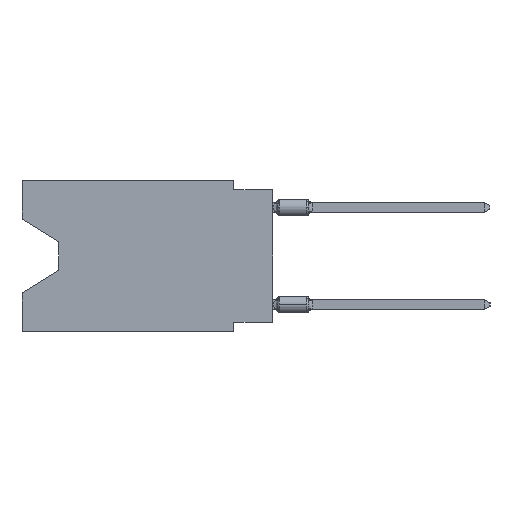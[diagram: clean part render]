
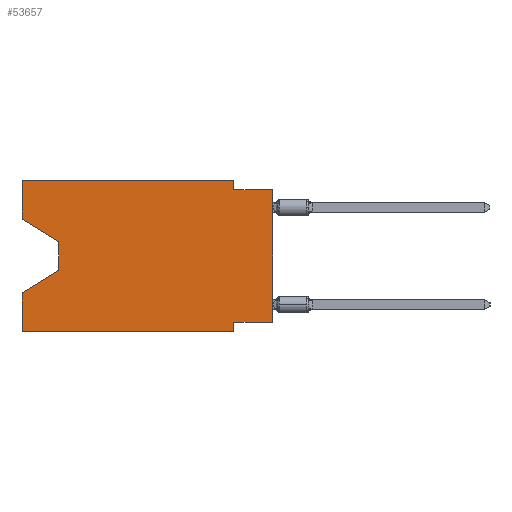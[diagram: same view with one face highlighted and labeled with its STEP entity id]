
A CAD part, left-side view. The second image highlights one B-rep face of the part: STEP entity #53657.
In plain terms, the highlighted planar face has unit normal (-1, 0, 0).
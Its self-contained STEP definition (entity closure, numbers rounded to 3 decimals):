
#431 = CARTESIAN_POINT ( 'NONE',  ( 0., 13.97, -5.893 ) ) ;
#1530 = LINE ( 'NONE', #18924, #46414 ) ;
#1816 = VECTOR ( 'NONE', #44940, 1000. ) ;
#2021 = EDGE_CURVE ( 'NONE', #47243, #37204, #41856, .T. ) ;
#2726 = LINE ( 'NONE', #46132, #11991 ) ;
#2740 = CARTESIAN_POINT ( 'NONE',  ( 0., 16.383, 0. ) ) ;
#3116 = CARTESIAN_POINT ( 'NONE',  ( 0., 0., -9.271 ) ) ;
#4385 = CARTESIAN_POINT ( 'NONE',  ( 0., 2.54, -9.271 ) ) ;
#5444 = EDGE_CURVE ( 'NONE', #17249, #12850, #1530, .T. ) ;
#7706 = CARTESIAN_POINT ( 'NONE',  ( 0., 0., -0.635 ) ) ;
#8406 = EDGE_CURVE ( 'NONE', #43531, #37204, #9874, .T. ) ;
#8539 = EDGE_CURVE ( 'NONE', #47243, #45560, #2726, .T. ) ;
#9874 = LINE ( 'NONE', #17868, #26458 ) ;
#9895 = AXIS2_PLACEMENT_3D ( 'NONE', #44052, #40604, #16307 ) ;
#10271 = VECTOR ( 'NONE', #11007, 1000. ) ;
#10964 = CARTESIAN_POINT ( 'NONE',  ( 0., 13.97, -4.013 ) ) ;
#11007 = DIRECTION ( 'NONE',  ( 0., -0.855, -0.519 ) ) ;
#11349 = DIRECTION ( 'NONE',  ( 0., 1., 0. ) ) ;
#11991 = VECTOR ( 'NONE', #24417, 1000. ) ;
#12544 = VECTOR ( 'NONE', #28981, 1000. ) ;
#12823 = DIRECTION ( 'NONE',  ( 0., 0., -1. ) ) ;
#12850 = VERTEX_POINT ( 'NONE', #21025 ) ;
#14395 = EDGE_CURVE ( 'NONE', #26433, #39106, #53634, .T. ) ;
#14722 = EDGE_CURVE ( 'NONE', #26433, #54521, #32077, .T. ) ;
#15387 = EDGE_CURVE ( 'NONE', #12850, #54521, #38267, .T. ) ;
#15642 = CARTESIAN_POINT ( 'NONE',  ( 0., 0., -9.271 ) ) ;
#16307 = DIRECTION ( 'NONE',  ( 0., 0., -1. ) ) ;
#16721 = VECTOR ( 'NONE', #23411, 1000. ) ;
#17249 = VERTEX_POINT ( 'NONE', #41831 ) ;
#17868 = CARTESIAN_POINT ( 'NONE',  ( 0., 13.97, -5.893 ) ) ;
#18774 = VECTOR ( 'NONE', #12823, 1000. ) ;
#18924 = CARTESIAN_POINT ( 'NONE',  ( 0., 2.54, 0. ) ) ;
#19131 = LINE ( 'NONE', #45983, #16721 ) ;
#20954 = EDGE_LOOP ( 'NONE', ( #41257, #39529, #29314, #48623, #48255, #26523, #36338, #36237, #52485, #49246, #40684, #54955 ) ) ;
#21025 = CARTESIAN_POINT ( 'NONE',  ( 0., 2.54, -0.635 ) ) ;
#21288 = CARTESIAN_POINT ( 'NONE',  ( 0., 13.97, -4.013 ) ) ;
#23183 = FACE_OUTER_BOUND ( 'NONE', #20954, .T. ) ;
#23394 = CARTESIAN_POINT ( 'NONE',  ( 0., 16.383, -9.906 ) ) ;
#23411 = DIRECTION ( 'NONE',  ( 0., 0., 1. ) ) ;
#23459 = VERTEX_POINT ( 'NONE', #49132 ) ;
#24336 = EDGE_CURVE ( 'NONE', #31201, #43531, #46089, .T. ) ;
#24417 = DIRECTION ( 'NONE',  ( 0., -1., 0. ) ) ;
#25396 = CARTESIAN_POINT ( 'NONE',  ( 0., 2.54, -9.906 ) ) ;
#25680 = LINE ( 'NONE', #25396, #18774 ) ;
#26433 = VERTEX_POINT ( 'NONE', #3116 ) ;
#26458 = VECTOR ( 'NONE', #31860, 1000. ) ;
#26523 = ORIENTED_EDGE ( 'NONE', *, *, #48307, .F. ) ;
#26979 = VECTOR ( 'NONE', #51761, 1000. ) ;
#27358 = VERTEX_POINT ( 'NONE', #38602 ) ;
#28981 = DIRECTION ( 'NONE',  ( 0., -1., 0. ) ) ;
#29261 = CARTESIAN_POINT ( 'NONE',  ( 0., 16.383, 0. ) ) ;
#29314 = ORIENTED_EDGE ( 'NONE', *, *, #8406, .T. ) ;
#29398 = DIRECTION ( 'NONE',  ( 0., -1., 0. ) ) ;
#31201 = VERTEX_POINT ( 'NONE', #21288 ) ;
#31860 = DIRECTION ( 'NONE',  ( 0., 0.855, -0.519 ) ) ;
#32077 = LINE ( 'NONE', #48920, #1816 ) ;
#33232 = DIRECTION ( 'NONE',  ( 0., 0., -1. ) ) ;
#34221 = EDGE_CURVE ( 'NONE', #23459, #17249, #42139, .T. ) ;
#35793 = DIRECTION ( 'NONE',  ( 0., 0., -1. ) ) ;
#36237 = ORIENTED_EDGE ( 'NONE', *, *, #14722, .T. ) ;
#36338 = ORIENTED_EDGE ( 'NONE', *, *, #14395, .F. ) ;
#36419 = VECTOR ( 'NONE', #11349, 1000. ) ;
#37204 = VERTEX_POINT ( 'NONE', #38518 ) ;
#38267 = LINE ( 'NONE', #7706, #43789 ) ;
#38518 = CARTESIAN_POINT ( 'NONE',  ( 0., 16.383, -7.36 ) ) ;
#38602 = CARTESIAN_POINT ( 'NONE',  ( 0., 16.383, -2.546 ) ) ;
#39106 = VERTEX_POINT ( 'NONE', #4385 ) ;
#39529 = ORIENTED_EDGE ( 'NONE', *, *, #24336, .T. ) ;
#39874 = EDGE_CURVE ( 'NONE', #27358, #23459, #19131, .T. ) ;
#40604 = DIRECTION ( 'NONE',  ( 1., 0., 0. ) ) ;
#40684 = ORIENTED_EDGE ( 'NONE', *, *, #34221, .F. ) ;
#40829 = EDGE_CURVE ( 'NONE', #27358, #31201, #41840, .T. ) ;
#40895 = PLANE ( 'NONE',  #9895 ) ;
#41257 = ORIENTED_EDGE ( 'NONE', *, *, #40829, .T. ) ;
#41580 = VECTOR ( 'NONE', #33232, 1000. ) ;
#41831 = CARTESIAN_POINT ( 'NONE',  ( 0., 2.54, 0. ) ) ;
#41840 = LINE ( 'NONE', #46407, #10271 ) ;
#41856 = LINE ( 'NONE', #2740, #26979 ) ;
#42139 = LINE ( 'NONE', #29261, #12544 ) ;
#43531 = VERTEX_POINT ( 'NONE', #431 ) ;
#43789 = VECTOR ( 'NONE', #29398, 1000. ) ;
#44052 = CARTESIAN_POINT ( 'NONE',  ( 0., 16.383, 0. ) ) ;
#44940 = DIRECTION ( 'NONE',  ( 0., 0., 1. ) ) ;
#45560 = VERTEX_POINT ( 'NONE', #49169 ) ;
#45983 = CARTESIAN_POINT ( 'NONE',  ( 0., 16.383, 0. ) ) ;
#46089 = LINE ( 'NONE', #10964, #41580 ) ;
#46132 = CARTESIAN_POINT ( 'NONE',  ( 0., 16.383, -9.906 ) ) ;
#46407 = CARTESIAN_POINT ( 'NONE',  ( 0., 16.383, -2.546 ) ) ;
#46414 = VECTOR ( 'NONE', #35793, 1000. ) ;
#47243 = VERTEX_POINT ( 'NONE', #23394 ) ;
#48255 = ORIENTED_EDGE ( 'NONE', *, *, #8539, .T. ) ;
#48307 = EDGE_CURVE ( 'NONE', #39106, #45560, #25680, .T. ) ;
#48623 = ORIENTED_EDGE ( 'NONE', *, *, #2021, .F. ) ;
#48920 = CARTESIAN_POINT ( 'NONE',  ( 0., 0., 0. ) ) ;
#49132 = CARTESIAN_POINT ( 'NONE',  ( 0., 16.383, 0. ) ) ;
#49169 = CARTESIAN_POINT ( 'NONE',  ( 0., 2.54, -9.906 ) ) ;
#49246 = ORIENTED_EDGE ( 'NONE', *, *, #5444, .F. ) ;
#50394 = CARTESIAN_POINT ( 'NONE',  ( 0., 0., -0.635 ) ) ;
#51761 = DIRECTION ( 'NONE',  ( 0., 0., 1. ) ) ;
#52485 = ORIENTED_EDGE ( 'NONE', *, *, #15387, .F. ) ;
#53634 = LINE ( 'NONE', #15642, #36419 ) ;
#53657 = ADVANCED_FACE ( 'NONE', ( #23183 ), #40895, .F. ) ;
#54521 = VERTEX_POINT ( 'NONE', #50394 ) ;
#54955 = ORIENTED_EDGE ( 'NONE', *, *, #39874, .F. ) ;
